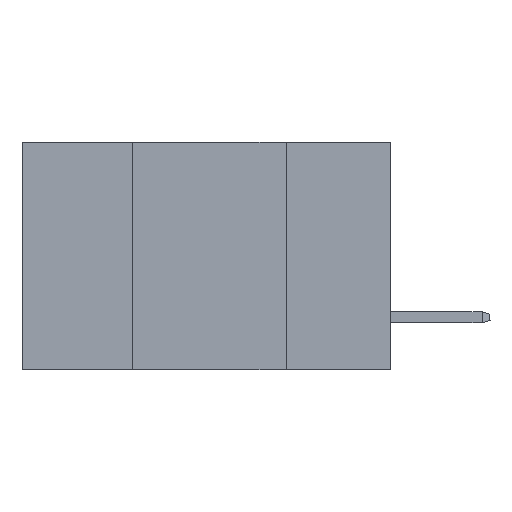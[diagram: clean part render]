
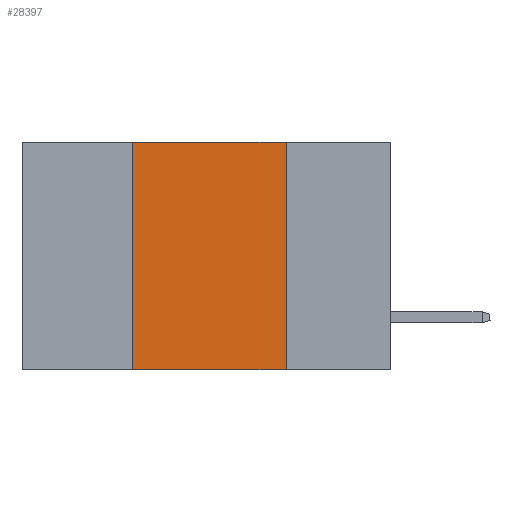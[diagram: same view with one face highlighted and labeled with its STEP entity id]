
A CAD part, left-side view. The second image highlights one B-rep face of the part: STEP entity #28397.
In plain terms, the highlighted planar face has unit normal (-1, 0, 0).
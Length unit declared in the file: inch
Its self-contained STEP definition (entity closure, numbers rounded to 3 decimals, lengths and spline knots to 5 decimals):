
#668 = EDGE_CURVE ( 'NONE', #11039, #26548, #6961, .T. ) ;
#1233 = VECTOR ( 'NONE', #1426, 39.37008 ) ;
#1426 = DIRECTION ( 'NONE',  ( 0., 0., -1. ) ) ;
#1617 = EDGE_CURVE ( 'NONE', #26548, #21627, #17443, .T. ) ;
#2971 = ORIENTED_EDGE ( 'NONE', *, *, #31540, .F. ) ;
#4378 = CARTESIAN_POINT ( 'NONE',  ( 0., 0.17, 0. ) ) ;
#5018 = CARTESIAN_POINT ( 'NONE',  ( 0., 0.42, -0.37 ) ) ;
#6340 = CARTESIAN_POINT ( 'NONE',  ( 0., 0.17, -0.37 ) ) ;
#6961 = LINE ( 'NONE', #15599, #23090 ) ;
#7142 = DIRECTION ( 'NONE',  ( 0., -1., 0. ) ) ;
#7447 = CARTESIAN_POINT ( 'NONE',  ( 0., 0.42, 0. ) ) ;
#8713 = CARTESIAN_POINT ( 'NONE',  ( 0., 0.42, 0. ) ) ;
#9429 = DIRECTION ( 'NONE',  ( 0., -1., 0. ) ) ;
#11039 = VERTEX_POINT ( 'NONE', #8713 ) ;
#12642 = VERTEX_POINT ( 'NONE', #5018 ) ;
#13065 = CARTESIAN_POINT ( 'NONE',  ( 0., 0.6, -0.37 ) ) ;
#15599 = CARTESIAN_POINT ( 'NONE',  ( 0., 0.6, 0. ) ) ;
#17443 = LINE ( 'NONE', #27803, #1233 ) ;
#18389 = VECTOR ( 'NONE', #9429, 39.37008 ) ;
#18410 = DIRECTION ( 'NONE',  ( 0., 0., -1. ) ) ;
#18585 = PLANE ( 'NONE',  #34318 ) ;
#20499 = ORIENTED_EDGE ( 'NONE', *, *, #668, .F. ) ;
#21048 = FACE_OUTER_BOUND ( 'NONE', #24680, .T. ) ;
#21627 = VERTEX_POINT ( 'NONE', #6340 ) ;
#23090 = VECTOR ( 'NONE', #7142, 39.37008 ) ;
#23451 = EDGE_CURVE ( 'NONE', #12642, #21627, #33502, .T. ) ;
#24680 = EDGE_LOOP ( 'NONE', ( #29670, #20499, #2971, #28216 ) ) ;
#26548 = VERTEX_POINT ( 'NONE', #4378 ) ;
#27803 = CARTESIAN_POINT ( 'NONE',  ( 0., 0.17, 0. ) ) ;
#28216 = ORIENTED_EDGE ( 'NONE', *, *, #23451, .T. ) ;
#28397 = ADVANCED_FACE ( 'NONE', ( #21048 ), #18585, .F. ) ;
#28899 = DIRECTION ( 'NONE',  ( 0., 0., 1. ) ) ;
#29670 = ORIENTED_EDGE ( 'NONE', *, *, #1617, .F. ) ;
#30515 = VECTOR ( 'NONE', #28899, 39.37008 ) ;
#31540 = EDGE_CURVE ( 'NONE', #12642, #11039, #31698, .T. ) ;
#31698 = LINE ( 'NONE', #7447, #30515 ) ;
#31742 = CARTESIAN_POINT ( 'NONE',  ( 0., 0.6, 0. ) ) ;
#32086 = DIRECTION ( 'NONE',  ( 1., 0., 0. ) ) ;
#33502 = LINE ( 'NONE', #13065, #18389 ) ;
#34318 = AXIS2_PLACEMENT_3D ( 'NONE', #31742, #32086, #18410 ) ;
